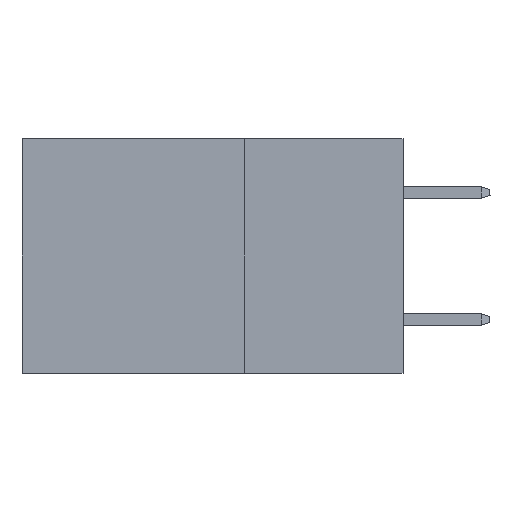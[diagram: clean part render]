
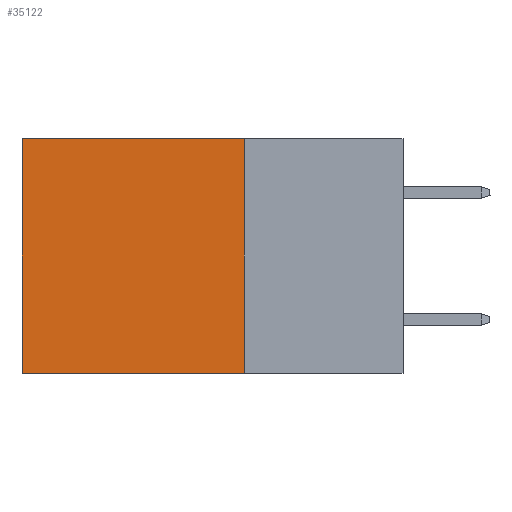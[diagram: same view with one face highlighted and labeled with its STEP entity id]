
A CAD part, left-side view. The second image highlights one B-rep face of the part: STEP entity #35122.
In plain terms, the highlighted planar face has unit normal (-1, 0, 0).
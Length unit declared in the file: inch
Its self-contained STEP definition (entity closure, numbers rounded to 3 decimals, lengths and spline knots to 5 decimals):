
#360 = DIRECTION ( 'NONE',  ( 0., 0., -1. ) ) ;
#821 = EDGE_CURVE ( 'NONE', #5660, #16066, #27566, .T. ) ;
#1213 = LINE ( 'NONE', #18514, #16601 ) ;
#2351 = EDGE_CURVE ( 'NONE', #23432, #9196, #21618, .T. ) ;
#2605 = EDGE_CURVE ( 'NONE', #5660, #23432, #1213, .T. ) ;
#3051 = PLANE ( 'NONE',  #36845 ) ;
#5660 = VERTEX_POINT ( 'NONE', #24035 ) ;
#6808 = ORIENTED_EDGE ( 'NONE', *, *, #9489, .F. ) ;
#7624 = CARTESIAN_POINT ( 'NONE',  ( 0.2875, 0.6, -0.37 ) ) ;
#9196 = VERTEX_POINT ( 'NONE', #7624 ) ;
#9314 = EDGE_LOOP ( 'NONE', ( #35124, #6808, #24740, #29741 ) ) ;
#9489 = EDGE_CURVE ( 'NONE', #16066, #9196, #27069, .T. ) ;
#10294 = VECTOR ( 'NONE', #17936, 39.37008 ) ;
#12095 = DIRECTION ( 'NONE',  ( 0., 1., 0. ) ) ;
#13293 = DIRECTION ( 'NONE',  ( 0., 0., -1. ) ) ;
#16066 = VERTEX_POINT ( 'NONE', #35872 ) ;
#16601 = VECTOR ( 'NONE', #12095, 39.37008 ) ;
#17105 = DIRECTION ( 'NONE',  ( 1., 0., 0. ) ) ;
#17725 = VECTOR ( 'NONE', #18648, 39.37008 ) ;
#17936 = DIRECTION ( 'NONE',  ( 0., 1., 0. ) ) ;
#18514 = CARTESIAN_POINT ( 'NONE',  ( 0.2875, 0.25, 0. ) ) ;
#18648 = DIRECTION ( 'NONE',  ( 0., 0., -1. ) ) ;
#18968 = CARTESIAN_POINT ( 'NONE',  ( 0.2875, 0.6, 0. ) ) ;
#21618 = LINE ( 'NONE', #18968, #32386 ) ;
#23392 = CARTESIAN_POINT ( 'NONE',  ( 0.2875, 0.25, 0. ) ) ;
#23432 = VERTEX_POINT ( 'NONE', #26092 ) ;
#24035 = CARTESIAN_POINT ( 'NONE',  ( 0.2875, 0.25, 0. ) ) ;
#24740 = ORIENTED_EDGE ( 'NONE', *, *, #821, .F. ) ;
#26092 = CARTESIAN_POINT ( 'NONE',  ( 0.2875, 0.6, 0. ) ) ;
#27069 = LINE ( 'NONE', #32762, #10294 ) ;
#27566 = LINE ( 'NONE', #33085, #17725 ) ;
#29288 = FACE_OUTER_BOUND ( 'NONE', #9314, .T. ) ;
#29741 = ORIENTED_EDGE ( 'NONE', *, *, #2605, .T. ) ;
#32386 = VECTOR ( 'NONE', #13293, 39.37008 ) ;
#32762 = CARTESIAN_POINT ( 'NONE',  ( 0.2875, 0.25, -0.37 ) ) ;
#33085 = CARTESIAN_POINT ( 'NONE',  ( 0.2875, 0.25, 0. ) ) ;
#35122 = ADVANCED_FACE ( 'NONE', ( #29288 ), #3051, .F. ) ;
#35124 = ORIENTED_EDGE ( 'NONE', *, *, #2351, .T. ) ;
#35872 = CARTESIAN_POINT ( 'NONE',  ( 0.2875, 0.25, -0.37 ) ) ;
#36845 = AXIS2_PLACEMENT_3D ( 'NONE', #23392, #17105, #360 ) ;
